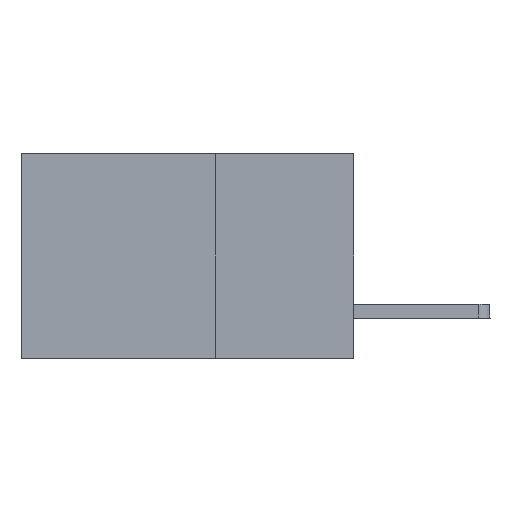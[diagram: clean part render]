
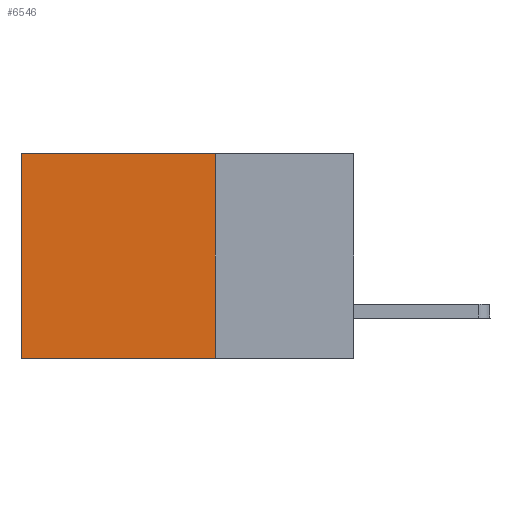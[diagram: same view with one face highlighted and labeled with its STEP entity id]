
A CAD part, left-side view. The second image highlights one B-rep face of the part: STEP entity #6546.
In plain terms, the highlighted planar face has unit normal (-1, 0, 0).
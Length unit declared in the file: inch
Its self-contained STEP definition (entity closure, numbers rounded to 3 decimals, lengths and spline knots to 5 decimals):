
#273 = CARTESIAN_POINT ( 'NONE',  ( 0.2875, 0.6, 0. ) ) ;
#516 = DIRECTION ( 'NONE',  ( 0., 1., 0. ) ) ;
#633 = CARTESIAN_POINT ( 'NONE',  ( 0.2875, 0.25, 0. ) ) ;
#866 = VECTOR ( 'NONE', #3724, 39.37008 ) ;
#1153 = ORIENTED_EDGE ( 'NONE', *, *, #3917, .T. ) ;
#1235 = ORIENTED_EDGE ( 'NONE', *, *, #7859, .F. ) ;
#1282 = LINE ( 'NONE', #6051, #866 ) ;
#1412 = ORIENTED_EDGE ( 'NONE', *, *, #4458, .F. ) ;
#1474 = ORIENTED_EDGE ( 'NONE', *, *, #5578, .T. ) ;
#1542 = LINE ( 'NONE', #4339, #7232 ) ;
#1583 = PLANE ( 'NONE',  #8130 ) ;
#2632 = VERTEX_POINT ( 'NONE', #6023 ) ;
#3106 = CARTESIAN_POINT ( 'NONE',  ( 0.2875, 0.6, -0.37 ) ) ;
#3693 = CARTESIAN_POINT ( 'NONE',  ( 0.2875, 0.25, 0. ) ) ;
#3724 = DIRECTION ( 'NONE',  ( 0., 1., 0. ) ) ;
#3902 = CARTESIAN_POINT ( 'NONE',  ( 0.2875, 0.25, 0. ) ) ;
#3917 = EDGE_CURVE ( 'NONE', #5603, #5420, #10025, .T. ) ;
#4218 = LINE ( 'NONE', #633, #9550 ) ;
#4339 = CARTESIAN_POINT ( 'NONE',  ( 0.2875, 0.25, 0. ) ) ;
#4458 = EDGE_CURVE ( 'NONE', #9684, #2632, #1542, .T. ) ;
#5112 = DIRECTION ( 'NONE',  ( 0., 0., -1. ) ) ;
#5420 = VERTEX_POINT ( 'NONE', #3106 ) ;
#5578 = EDGE_CURVE ( 'NONE', #9684, #5603, #4218, .T. ) ;
#5603 = VERTEX_POINT ( 'NONE', #273 ) ;
#5639 = DIRECTION ( 'NONE',  ( 0., 0., -1. ) ) ;
#6023 = CARTESIAN_POINT ( 'NONE',  ( 0.2875, 0.25, -0.37 ) ) ;
#6051 = CARTESIAN_POINT ( 'NONE',  ( 0.2875, 0.25, -0.37 ) ) ;
#6546 = ADVANCED_FACE ( 'NONE', ( #6994 ), #1583, .F. ) ;
#6994 = FACE_OUTER_BOUND ( 'NONE', #10508, .T. ) ;
#7232 = VECTOR ( 'NONE', #5639, 39.37008 ) ;
#7384 = VECTOR ( 'NONE', #10287, 39.37008 ) ;
#7859 = EDGE_CURVE ( 'NONE', #2632, #5420, #1282, .T. ) ;
#8130 = AXIS2_PLACEMENT_3D ( 'NONE', #3902, #11224, #5112 ) ;
#9550 = VECTOR ( 'NONE', #516, 39.37008 ) ;
#9684 = VERTEX_POINT ( 'NONE', #3693 ) ;
#10025 = LINE ( 'NONE', #10145, #7384 ) ;
#10145 = CARTESIAN_POINT ( 'NONE',  ( 0.2875, 0.6, 0. ) ) ;
#10287 = DIRECTION ( 'NONE',  ( 0., 0., -1. ) ) ;
#10508 = EDGE_LOOP ( 'NONE', ( #1153, #1235, #1412, #1474 ) ) ;
#11224 = DIRECTION ( 'NONE',  ( 1., 0., 0. ) ) ;
